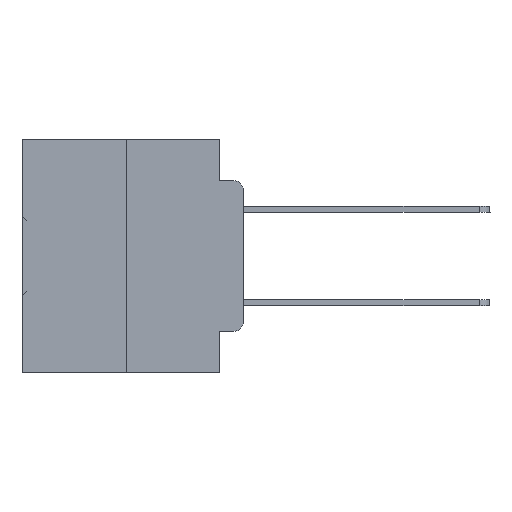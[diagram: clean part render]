
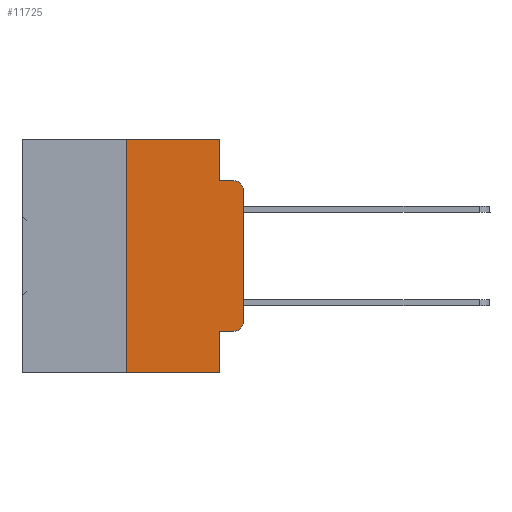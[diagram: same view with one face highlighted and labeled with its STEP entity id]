
A CAD part, left-side view. The second image highlights one B-rep face of the part: STEP entity #11725.
In plain terms, the highlighted planar face has unit normal (-1, 0, 0).
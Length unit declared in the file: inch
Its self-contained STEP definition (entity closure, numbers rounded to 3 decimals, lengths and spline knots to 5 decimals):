
#29 = ORIENTED_EDGE ( 'NONE', *, *, #23705, .F. ) ;
#1027 = ORIENTED_EDGE ( 'NONE', *, *, #7916, .F. ) ;
#1056 = VERTEX_POINT ( 'NONE', #37936 ) ;
#1635 = DIRECTION ( 'NONE',  ( 0., 0., 1. ) ) ;
#1744 = LINE ( 'NONE', #14968, #35921 ) ;
#1759 = AXIS2_PLACEMENT_3D ( 'NONE', #2704, #14693, #35869 ) ;
#1902 = CARTESIAN_POINT ( 'NONE',  ( 0., 0.25, 0. ) ) ;
#2704 = CARTESIAN_POINT ( 'NONE',  ( 0., 0.02, -0.1085 ) ) ;
#2819 = ORIENTED_EDGE ( 'NONE', *, *, #5045, .F. ) ;
#2980 = CARTESIAN_POINT ( 'NONE',  ( 0., 0., -0.3915 ) ) ;
#3207 = VERTEX_POINT ( 'NONE', #2980 ) ;
#4276 = CARTESIAN_POINT ( 'NONE',  ( 0., 0.473, 0. ) ) ;
#4381 = CARTESIAN_POINT ( 'NONE',  ( 0., 0.02, -0.0885 ) ) ;
#4486 = VECTOR ( 'NONE', #13450, 39.37008 ) ;
#5045 = EDGE_CURVE ( 'NONE', #19324, #1056, #28715, .T. ) ;
#6448 = VECTOR ( 'NONE', #35111, 39.37008 ) ;
#6524 = DIRECTION ( 'NONE',  ( -1., 0., 0. ) ) ;
#6799 = EDGE_CURVE ( 'NONE', #16128, #10001, #35532, .T. ) ;
#7048 = DIRECTION ( 'NONE',  ( 0., 0., -1. ) ) ;
#7726 = VECTOR ( 'NONE', #15613, 39.37008 ) ;
#7916 = EDGE_CURVE ( 'NONE', #10434, #19034, #32595, .T. ) ;
#8260 = ORIENTED_EDGE ( 'NONE', *, *, #17966, .F. ) ;
#8331 = LINE ( 'NONE', #9844, #37742 ) ;
#8859 = EDGE_CURVE ( 'NONE', #37575, #19034, #38188, .T. ) ;
#9332 = DIRECTION ( 'NONE',  ( 0., 0., -1. ) ) ;
#9844 = CARTESIAN_POINT ( 'NONE',  ( 0., 0.473, -0.5 ) ) ;
#10001 = VERTEX_POINT ( 'NONE', #26269 ) ;
#10434 = VERTEX_POINT ( 'NONE', #31268 ) ;
#11618 = EDGE_CURVE ( 'NONE', #3207, #37575, #23770, .T. ) ;
#11725 = ADVANCED_FACE ( 'NONE', ( #32266 ), #22624, .F. ) ;
#12571 = EDGE_CURVE ( 'NONE', #16128, #20687, #1744, .T. ) ;
#13014 = DIRECTION ( 'NONE',  ( 0., -1., 0. ) ) ;
#13450 = DIRECTION ( 'NONE',  ( 0., -1., 0. ) ) ;
#14205 = VECTOR ( 'NONE', #15380, 39.37008 ) ;
#14431 = EDGE_CURVE ( 'NONE', #22113, #20687, #8331, .T. ) ;
#14693 = DIRECTION ( 'NONE',  ( -1., 0., 0. ) ) ;
#14968 = CARTESIAN_POINT ( 'NONE',  ( 0., 0.051, 0. ) ) ;
#15247 = ORIENTED_EDGE ( 'NONE', *, *, #29092, .T. ) ;
#15380 = DIRECTION ( 'NONE',  ( 0., -1., 0. ) ) ;
#15613 = DIRECTION ( 'NONE',  ( 0., 0., -1. ) ) ;
#15772 = CARTESIAN_POINT ( 'NONE',  ( 0., 0., -0.1085 ) ) ;
#16128 = VERTEX_POINT ( 'NONE', #29380 ) ;
#16331 = CARTESIAN_POINT ( 'NONE',  ( 0., 0.051, -0.5 ) ) ;
#17966 = EDGE_CURVE ( 'NONE', #1056, #10434, #21062, .T. ) ;
#19034 = VERTEX_POINT ( 'NONE', #4381 ) ;
#19324 = VERTEX_POINT ( 'NONE', #1902 ) ;
#20687 = VERTEX_POINT ( 'NONE', #16331 ) ;
#20953 = DIRECTION ( 'NONE',  ( 0., 0., -1. ) ) ;
#21062 = LINE ( 'NONE', #24902, #7726 ) ;
#21616 = CARTESIAN_POINT ( 'NONE',  ( 0., 0.051, -0.4115 ) ) ;
#21838 = VECTOR ( 'NONE', #1635, 39.37008 ) ;
#21938 = CARTESIAN_POINT ( 'NONE',  ( 0., 0.25, -0.5 ) ) ;
#22113 = VERTEX_POINT ( 'NONE', #21938 ) ;
#22624 = PLANE ( 'NONE',  #31888 ) ;
#22822 = CIRCLE ( 'NONE', #24714, 0.02 ) ;
#23705 = EDGE_CURVE ( 'NONE', #22113, #19324, #35144, .T. ) ;
#23770 = LINE ( 'NONE', #35075, #21838 ) ;
#24714 = AXIS2_PLACEMENT_3D ( 'NONE', #24748, #6524, #9332 ) ;
#24748 = CARTESIAN_POINT ( 'NONE',  ( 0., 0.02, -0.3915 ) ) ;
#24902 = CARTESIAN_POINT ( 'NONE',  ( 0., 0.051, 0. ) ) ;
#25857 = CARTESIAN_POINT ( 'NONE',  ( 0., 0.051, -0.0885 ) ) ;
#26269 = CARTESIAN_POINT ( 'NONE',  ( 0., 0.02, -0.4115 ) ) ;
#28715 = LINE ( 'NONE', #28855, #4486 ) ;
#28855 = CARTESIAN_POINT ( 'NONE',  ( 0., 0.473, 0. ) ) ;
#28988 = ORIENTED_EDGE ( 'NONE', *, *, #11618, .T. ) ;
#29092 = EDGE_CURVE ( 'NONE', #10001, #3207, #22822, .T. ) ;
#29380 = CARTESIAN_POINT ( 'NONE',  ( 0., 0.051, -0.4115 ) ) ;
#30716 = ORIENTED_EDGE ( 'NONE', *, *, #14431, .T. ) ;
#31268 = CARTESIAN_POINT ( 'NONE',  ( 0., 0.051, -0.0885 ) ) ;
#31888 = AXIS2_PLACEMENT_3D ( 'NONE', #4276, #37169, #7048 ) ;
#32266 = FACE_OUTER_BOUND ( 'NONE', #36591, .T. ) ;
#32595 = LINE ( 'NONE', #25857, #6448 ) ;
#35075 = CARTESIAN_POINT ( 'NONE',  ( 0., 0., 0. ) ) ;
#35111 = DIRECTION ( 'NONE',  ( 0., -1., 0. ) ) ;
#35144 = LINE ( 'NONE', #38941, #37977 ) ;
#35266 = ORIENTED_EDGE ( 'NONE', *, *, #6799, .T. ) ;
#35530 = DIRECTION ( 'NONE',  ( 0., 0., 1. ) ) ;
#35532 = LINE ( 'NONE', #21616, #14205 ) ;
#35869 = DIRECTION ( 'NONE',  ( 0., 0., -1. ) ) ;
#35921 = VECTOR ( 'NONE', #20953, 39.37008 ) ;
#36222 = ORIENTED_EDGE ( 'NONE', *, *, #12571, .F. ) ;
#36591 = EDGE_LOOP ( 'NONE', ( #28988, #37041, #1027, #8260, #2819, #29, #30716, #36222, #35266, #15247 ) ) ;
#37041 = ORIENTED_EDGE ( 'NONE', *, *, #8859, .T. ) ;
#37169 = DIRECTION ( 'NONE',  ( 1., 0., 0. ) ) ;
#37575 = VERTEX_POINT ( 'NONE', #15772 ) ;
#37742 = VECTOR ( 'NONE', #13014, 39.37008 ) ;
#37936 = CARTESIAN_POINT ( 'NONE',  ( 0., 0.051, 0. ) ) ;
#37977 = VECTOR ( 'NONE', #35530, 39.37008 ) ;
#38188 = CIRCLE ( 'NONE', #1759, 0.02 ) ;
#38941 = CARTESIAN_POINT ( 'NONE',  ( 0., 0.25, 0. ) ) ;
